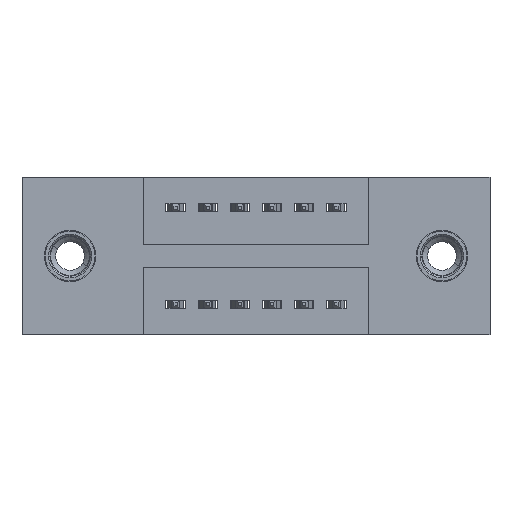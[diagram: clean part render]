
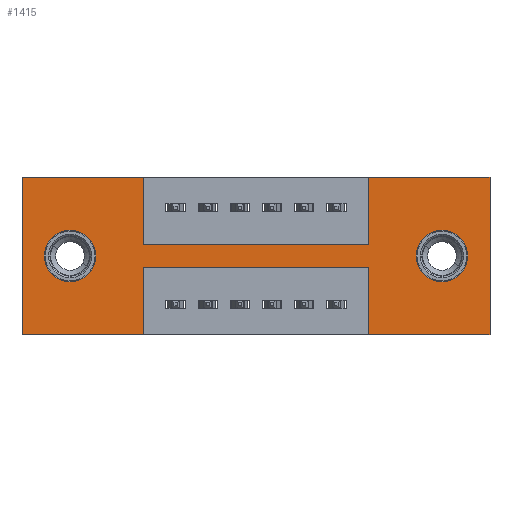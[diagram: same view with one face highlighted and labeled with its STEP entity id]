
A CAD part, front view. The second image highlights one B-rep face of the part: STEP entity #1415.
In plain terms, the highlighted planar face has unit normal (0, -1, 0).
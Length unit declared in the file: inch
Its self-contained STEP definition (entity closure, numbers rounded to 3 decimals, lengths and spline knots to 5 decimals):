
#17 = ORIENTED_EDGE ( 'NONE', *, *, #8628, .F. ) ;
#27 = VERTEX_POINT ( 'NONE', #7843 ) ;
#30 = CARTESIAN_POINT ( 'NONE',  ( 0.3775, 0., -0.49 ) ) ;
#56 = ORIENTED_EDGE ( 'NONE', *, *, #9000, .F. ) ;
#257 = ORIENTED_EDGE ( 'NONE', *, *, #8767, .F. ) ;
#367 = LINE ( 'NONE', #6275, #4242 ) ;
#369 = VERTEX_POINT ( 'NONE', #8981 ) ;
#375 = LINE ( 'NONE', #7995, #4373 ) ;
#606 = EDGE_LOOP ( 'NONE', ( #2022, #17, #2317, #257, #1225, #2949, #2294, #6311, #6599, #6043, #56, #2867 ) ) ;
#631 = DIRECTION ( 'NONE',  ( -1., 0., 0. ) ) ;
#773 = EDGE_CURVE ( 'NONE', #8387, #6136, #5053, .T. ) ;
#823 = CARTESIAN_POINT ( 'NONE',  ( 0.1495, 0., -0.165 ) ) ;
#836 = DIRECTION ( 'NONE',  ( 0., 1., 0. ) ) ;
#909 = FACE_OUTER_BOUND ( 'NONE', #606, .T. ) ;
#1110 = CARTESIAN_POINT ( 'NONE',  ( 0.3775, 0., -0.28 ) ) ;
#1140 = FACE_BOUND ( 'NONE', #8272, .T. ) ;
#1171 = LINE ( 'NONE', #8231, #1634 ) ;
#1225 = ORIENTED_EDGE ( 'NONE', *, *, #4101, .F. ) ;
#1415 = ADVANCED_FACE ( 'NONE', ( #8696, #1140, #909 ), #8529, .T. ) ;
#1444 = VERTEX_POINT ( 'NONE', #1110 ) ;
#1490 = CARTESIAN_POINT ( 'NONE',  ( 1.3055, 0., -0.245 ) ) ;
#1541 = VERTEX_POINT ( 'NONE', #6647 ) ;
#1542 = DIRECTION ( 'NONE',  ( 0., 0., 1. ) ) ;
#1634 = VECTOR ( 'NONE', #3699, 39.37008 ) ;
#1692 = EDGE_CURVE ( 'NONE', #2953, #1541, #8086, .T. ) ;
#1761 = DIRECTION ( 'NONE',  ( 1., 0., 0. ) ) ;
#1859 = ORIENTED_EDGE ( 'NONE', *, *, #5895, .T. ) ;
#1900 = DIRECTION ( 'NONE',  ( 1., 0., 0. ) ) ;
#1922 = VERTEX_POINT ( 'NONE', #2370 ) ;
#1934 = VERTEX_POINT ( 'NONE', #9143 ) ;
#1986 = DIRECTION ( 'NONE',  ( 0., 0., 1. ) ) ;
#2009 = LINE ( 'NONE', #2084, #7557 ) ;
#2013 = CARTESIAN_POINT ( 'NONE',  ( 1.455, 0., -0.49 ) ) ;
#2019 = CARTESIAN_POINT ( 'NONE',  ( 0.1495, 0., -0.245 ) ) ;
#2022 = ORIENTED_EDGE ( 'NONE', *, *, #6621, .F. ) ;
#2084 = CARTESIAN_POINT ( 'NONE',  ( 0.3775, 0., -0.21 ) ) ;
#2095 = LINE ( 'NONE', #3855, #6839 ) ;
#2294 = ORIENTED_EDGE ( 'NONE', *, *, #9742, .F. ) ;
#2315 = DIRECTION ( 'NONE',  ( 0., 1., 0. ) ) ;
#2317 = ORIENTED_EDGE ( 'NONE', *, *, #3182, .F. ) ;
#2370 = CARTESIAN_POINT ( 'NONE',  ( 0.3775, 0., -0.21 ) ) ;
#2779 = EDGE_CURVE ( 'NONE', #8205, #2953, #375, .T. ) ;
#2832 = DIRECTION ( 'NONE',  ( 0., 0., -1. ) ) ;
#2867 = ORIENTED_EDGE ( 'NONE', *, *, #3230, .F. ) ;
#2949 = ORIENTED_EDGE ( 'NONE', *, *, #3792, .F. ) ;
#2953 = VERTEX_POINT ( 'NONE', #3750 ) ;
#3102 = CARTESIAN_POINT ( 'NONE',  ( 0., 0., 0. ) ) ;
#3127 = VECTOR ( 'NONE', #1542, 39.37008 ) ;
#3166 = CIRCLE ( 'NONE', #3746, 0.08 ) ;
#3182 = EDGE_CURVE ( 'NONE', #9276, #1922, #2009, .T. ) ;
#3230 = EDGE_CURVE ( 'NONE', #4606, #369, #8498, .T. ) ;
#3274 = CARTESIAN_POINT ( 'NONE',  ( 0.1495, 0., -0.325 ) ) ;
#3464 = CARTESIAN_POINT ( 'NONE',  ( 1.0775, 0., 0. ) ) ;
#3699 = DIRECTION ( 'NONE',  ( 0., 0., -1. ) ) ;
#3724 = DIRECTION ( 'NONE',  ( 0., 0., -1. ) ) ;
#3746 = AXIS2_PLACEMENT_3D ( 'NONE', #4576, #836, #4613 ) ;
#3750 = CARTESIAN_POINT ( 'NONE',  ( 1.0775, 0., -0.49 ) ) ;
#3792 = EDGE_CURVE ( 'NONE', #3918, #1934, #4469, .T. ) ;
#3855 = CARTESIAN_POINT ( 'NONE',  ( 0., 0., 0. ) ) ;
#3918 = VERTEX_POINT ( 'NONE', #30 ) ;
#4019 = VERTEX_POINT ( 'NONE', #5999 ) ;
#4101 = EDGE_CURVE ( 'NONE', #1934, #4019, #2095, .T. ) ;
#4242 = VECTOR ( 'NONE', #1761, 39.37008 ) ;
#4299 = LINE ( 'NONE', #5992, #3127 ) ;
#4373 = VECTOR ( 'NONE', #6458, 39.37008 ) ;
#4469 = LINE ( 'NONE', #5925, #4843 ) ;
#4576 = CARTESIAN_POINT ( 'NONE',  ( 0.1495, 0., -0.245 ) ) ;
#4606 = VERTEX_POINT ( 'NONE', #3464 ) ;
#4613 = DIRECTION ( 'NONE',  ( 0., 0., 1. ) ) ;
#4843 = VECTOR ( 'NONE', #631, 39.37008 ) ;
#4868 = DIRECTION ( 'NONE',  ( 0., 0., 1. ) ) ;
#4931 = CIRCLE ( 'NONE', #9532, 0.08 ) ;
#5053 = CIRCLE ( 'NONE', #7054, 0.08 ) ;
#5291 = DIRECTION ( 'NONE',  ( -1., 0., 0. ) ) ;
#5620 = CIRCLE ( 'NONE', #9599, 0.08 ) ;
#5685 = VECTOR ( 'NONE', #9743, 39.37008 ) ;
#5804 = ORIENTED_EDGE ( 'NONE', *, *, #773, .T. ) ;
#5869 = VECTOR ( 'NONE', #4868, 39.37008 ) ;
#5895 = EDGE_CURVE ( 'NONE', #7386, #7849, #4931, .T. ) ;
#5925 = CARTESIAN_POINT ( 'NONE',  ( 0., 0., -0.49 ) ) ;
#5992 = CARTESIAN_POINT ( 'NONE',  ( 1.0775, 0., -0.21 ) ) ;
#5999 = CARTESIAN_POINT ( 'NONE',  ( 0., 0., 0. ) ) ;
#6043 = ORIENTED_EDGE ( 'NONE', *, *, #2779, .F. ) ;
#6096 = CARTESIAN_POINT ( 'NONE',  ( 0.3775, 0., -0.28 ) ) ;
#6136 = VERTEX_POINT ( 'NONE', #6356 ) ;
#6275 = CARTESIAN_POINT ( 'NONE',  ( 0.3775, 0., -0.21 ) ) ;
#6311 = ORIENTED_EDGE ( 'NONE', *, *, #8368, .F. ) ;
#6329 = CARTESIAN_POINT ( 'NONE',  ( 0.3775, 0., 0. ) ) ;
#6356 = CARTESIAN_POINT ( 'NONE',  ( 1.3055, 0., -0.165 ) ) ;
#6458 = DIRECTION ( 'NONE',  ( -1., 0., 0. ) ) ;
#6499 = VECTOR ( 'NONE', #1900, 39.37008 ) ;
#6599 = ORIENTED_EDGE ( 'NONE', *, *, #1692, .F. ) ;
#6606 = CARTESIAN_POINT ( 'NONE',  ( 1.0775, 0., -0.28 ) ) ;
#6621 = EDGE_CURVE ( 'NONE', #27, #4606, #4299, .T. ) ;
#6647 = CARTESIAN_POINT ( 'NONE',  ( 1.0775, 0., -0.28 ) ) ;
#6801 = CARTESIAN_POINT ( 'NONE',  ( 0.3775, 0., -0.28 ) ) ;
#6839 = VECTOR ( 'NONE', #8415, 39.37008 ) ;
#6987 = EDGE_CURVE ( 'NONE', #6136, #8387, #5620, .T. ) ;
#7054 = AXIS2_PLACEMENT_3D ( 'NONE', #1490, #2315, #7595 ) ;
#7107 = DIRECTION ( 'NONE',  ( 0., 0., -1. ) ) ;
#7296 = VECTOR ( 'NONE', #3724, 39.37008 ) ;
#7317 = LINE ( 'NONE', #8047, #6499 ) ;
#7322 = CARTESIAN_POINT ( 'NONE',  ( 1.3055, 0., -0.245 ) ) ;
#7386 = VERTEX_POINT ( 'NONE', #3274 ) ;
#7486 = CARTESIAN_POINT ( 'NONE',  ( 1.3055, 0., -0.325 ) ) ;
#7557 = VECTOR ( 'NONE', #9709, 39.37008 ) ;
#7595 = DIRECTION ( 'NONE',  ( 0., 0., -1. ) ) ;
#7768 = CARTESIAN_POINT ( 'NONE',  ( 0., 0., -0.49 ) ) ;
#7819 = AXIS2_PLACEMENT_3D ( 'NONE', #7768, #8637, #7107 ) ;
#7843 = CARTESIAN_POINT ( 'NONE',  ( 1.0775, 0., -0.21 ) ) ;
#7849 = VERTEX_POINT ( 'NONE', #823 ) ;
#7995 = CARTESIAN_POINT ( 'NONE',  ( 0., 0., -0.49 ) ) ;
#8047 = CARTESIAN_POINT ( 'NONE',  ( 0., 0., 0. ) ) ;
#8060 = DIRECTION ( 'NONE',  ( 0., 1., 0. ) ) ;
#8086 = LINE ( 'NONE', #6606, #5869 ) ;
#8205 = VERTEX_POINT ( 'NONE', #2013 ) ;
#8231 = CARTESIAN_POINT ( 'NONE',  ( 1.455, 0., 0. ) ) ;
#8272 = EDGE_LOOP ( 'NONE', ( #8624, #1859 ) ) ;
#8368 = EDGE_CURVE ( 'NONE', #1541, #1444, #9068, .T. ) ;
#8387 = VERTEX_POINT ( 'NONE', #7486 ) ;
#8415 = DIRECTION ( 'NONE',  ( 0., 0., 1. ) ) ;
#8498 = LINE ( 'NONE', #3102, #5685 ) ;
#8529 = PLANE ( 'NONE',  #7819 ) ;
#8624 = ORIENTED_EDGE ( 'NONE', *, *, #8971, .T. ) ;
#8628 = EDGE_CURVE ( 'NONE', #1922, #27, #367, .T. ) ;
#8637 = DIRECTION ( 'NONE',  ( 0., -1., 0. ) ) ;
#8696 = FACE_BOUND ( 'NONE', #8785, .T. ) ;
#8767 = EDGE_CURVE ( 'NONE', #4019, #9276, #7317, .T. ) ;
#8785 = EDGE_LOOP ( 'NONE', ( #9682, #5804 ) ) ;
#8832 = DIRECTION ( 'NONE',  ( 0., 1., 0. ) ) ;
#8971 = EDGE_CURVE ( 'NONE', #7849, #7386, #3166, .T. ) ;
#8981 = CARTESIAN_POINT ( 'NONE',  ( 1.455, 0., 0. ) ) ;
#9000 = EDGE_CURVE ( 'NONE', #369, #8205, #1171, .T. ) ;
#9068 = LINE ( 'NONE', #6801, #9411 ) ;
#9143 = CARTESIAN_POINT ( 'NONE',  ( 0., 0., -0.49 ) ) ;
#9146 = LINE ( 'NONE', #6096, #7296 ) ;
#9276 = VERTEX_POINT ( 'NONE', #6329 ) ;
#9411 = VECTOR ( 'NONE', #5291, 39.37008 ) ;
#9532 = AXIS2_PLACEMENT_3D ( 'NONE', #2019, #8060, #1986 ) ;
#9599 = AXIS2_PLACEMENT_3D ( 'NONE', #7322, #8832, #2832 ) ;
#9682 = ORIENTED_EDGE ( 'NONE', *, *, #6987, .T. ) ;
#9709 = DIRECTION ( 'NONE',  ( 0., 0., -1. ) ) ;
#9742 = EDGE_CURVE ( 'NONE', #1444, #3918, #9146, .T. ) ;
#9743 = DIRECTION ( 'NONE',  ( 1., 0., 0. ) ) ;
